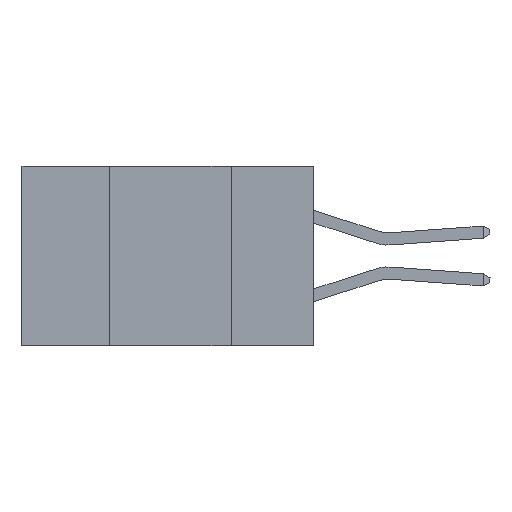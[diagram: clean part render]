
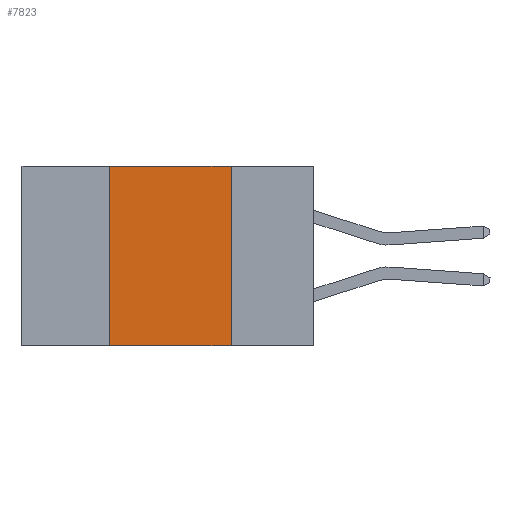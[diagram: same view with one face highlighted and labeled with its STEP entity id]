
A CAD part, left-side view. The second image highlights one B-rep face of the part: STEP entity #7823.
In plain terms, the highlighted planar face has unit normal (-1, 0, 0).
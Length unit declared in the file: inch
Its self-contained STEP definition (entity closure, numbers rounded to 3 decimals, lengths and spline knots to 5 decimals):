
#852 = EDGE_CURVE ( 'NONE', #14349, #16020, #16222, .T. ) ;
#978 = ORIENTED_EDGE ( 'NONE', *, *, #852, .T. ) ;
#1238 = EDGE_CURVE ( 'NONE', #14349, #9189, #10145, .T. ) ;
#1530 = CARTESIAN_POINT ( 'NONE',  ( 0., 0.17, 0. ) ) ;
#1820 = FACE_OUTER_BOUND ( 'NONE', #15115, .T. ) ;
#2423 = CARTESIAN_POINT ( 'NONE',  ( 0., 0.42, -0.37 ) ) ;
#2484 = ORIENTED_EDGE ( 'NONE', *, *, #3187, .F. ) ;
#2645 = ORIENTED_EDGE ( 'NONE', *, *, #16957, .F. ) ;
#3187 = EDGE_CURVE ( 'NONE', #9189, #8139, #4205, .T. ) ;
#3515 = ORIENTED_EDGE ( 'NONE', *, *, #1238, .F. ) ;
#4205 = LINE ( 'NONE', #9129, #15175 ) ;
#5237 = CARTESIAN_POINT ( 'NONE',  ( 0., 0.17, -0.37 ) ) ;
#5414 = VECTOR ( 'NONE', #13548, 39.37008 ) ;
#5791 = CARTESIAN_POINT ( 'NONE',  ( 0., 0.6, 0. ) ) ;
#5888 = CARTESIAN_POINT ( 'NONE',  ( 0., 0.42, 0. ) ) ;
#7308 = DIRECTION ( 'NONE',  ( 0., 0., -1. ) ) ;
#7823 = ADVANCED_FACE ( 'NONE', ( #1820 ), #19142, .F. ) ;
#8139 = VERTEX_POINT ( 'NONE', #16920 ) ;
#9013 = DIRECTION ( 'NONE',  ( 0., -1., 0. ) ) ;
#9129 = CARTESIAN_POINT ( 'NONE',  ( 0., 0.6, 0. ) ) ;
#9189 = VERTEX_POINT ( 'NONE', #5888 ) ;
#9680 = VECTOR ( 'NONE', #18048, 39.37008 ) ;
#10145 = LINE ( 'NONE', #16549, #9680 ) ;
#11579 = DIRECTION ( 'NONE',  ( 0., -1., 0. ) ) ;
#12239 = VECTOR ( 'NONE', #11579, 39.37008 ) ;
#13548 = DIRECTION ( 'NONE',  ( 0., 0., -1. ) ) ;
#13797 = LINE ( 'NONE', #1530, #5414 ) ;
#14349 = VERTEX_POINT ( 'NONE', #2423 ) ;
#15115 = EDGE_LOOP ( 'NONE', ( #2645, #2484, #3515, #978 ) ) ;
#15175 = VECTOR ( 'NONE', #9013, 39.37008 ) ;
#15216 = CARTESIAN_POINT ( 'NONE',  ( 0., 0.6, -0.37 ) ) ;
#16020 = VERTEX_POINT ( 'NONE', #5237 ) ;
#16217 = DIRECTION ( 'NONE',  ( 1., 0., 0. ) ) ;
#16222 = LINE ( 'NONE', #15216, #12239 ) ;
#16549 = CARTESIAN_POINT ( 'NONE',  ( 0., 0.42, 0. ) ) ;
#16920 = CARTESIAN_POINT ( 'NONE',  ( 0., 0.17, 0. ) ) ;
#16957 = EDGE_CURVE ( 'NONE', #8139, #16020, #13797, .T. ) ;
#17206 = AXIS2_PLACEMENT_3D ( 'NONE', #5791, #16217, #7308 ) ;
#18048 = DIRECTION ( 'NONE',  ( 0., 0., 1. ) ) ;
#19142 = PLANE ( 'NONE',  #17206 ) ;
